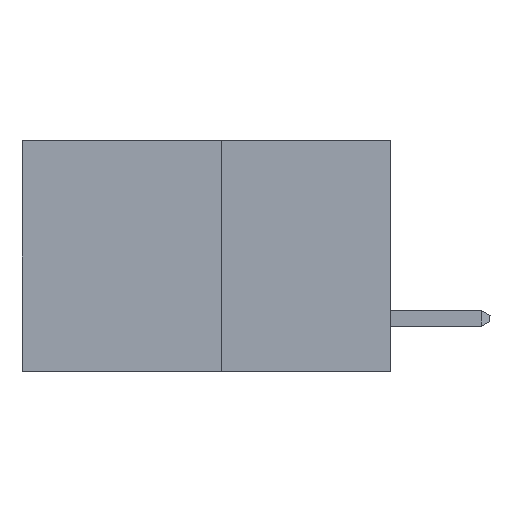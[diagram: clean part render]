
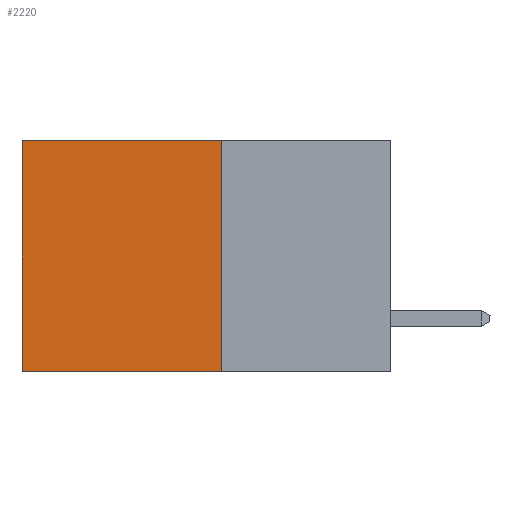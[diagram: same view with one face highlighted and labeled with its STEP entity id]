
A CAD part, left-side view. The second image highlights one B-rep face of the part: STEP entity #2220.
In plain terms, the highlighted planar face has unit normal (-1, 0, 0).
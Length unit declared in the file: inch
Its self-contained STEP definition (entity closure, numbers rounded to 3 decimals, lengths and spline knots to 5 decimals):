
#460 = DIRECTION ( 'NONE',  ( 1., 0., 0. ) ) ;
#852 = FACE_OUTER_BOUND ( 'NONE', #5256, .T. ) ;
#894 = EDGE_CURVE ( 'NONE', #5952, #5302, #2677, .T. ) ;
#1231 = CARTESIAN_POINT ( 'NONE',  ( 0.277, 0.59, -0.37 ) ) ;
#1289 = CARTESIAN_POINT ( 'NONE',  ( 0.277, 0.27, -0.37 ) ) ;
#1688 = EDGE_CURVE ( 'NONE', #5302, #4373, #8798, .T. ) ;
#1799 = ORIENTED_EDGE ( 'NONE', *, *, #894, .F. ) ;
#1964 = DIRECTION ( 'NONE',  ( 0., 1., 0. ) ) ;
#2111 = VECTOR ( 'NONE', #2915, 39.37008 ) ;
#2211 = CARTESIAN_POINT ( 'NONE',  ( 0.277, 0.27, 0. ) ) ;
#2220 = ADVANCED_FACE ( 'NONE', ( #852 ), #3283, .F. ) ;
#2549 = CARTESIAN_POINT ( 'NONE',  ( 0.277, 0.59, -0.37 ) ) ;
#2677 = LINE ( 'NONE', #3912, #8104 ) ;
#2915 = DIRECTION ( 'NONE',  ( 0., 1., 0. ) ) ;
#3283 = PLANE ( 'NONE',  #5911 ) ;
#3548 = VERTEX_POINT ( 'NONE', #8584 ) ;
#3601 = VECTOR ( 'NONE', #1964, 39.37008 ) ;
#3861 = CARTESIAN_POINT ( 'NONE',  ( 0.277, 0.27, -0.37 ) ) ;
#3912 = CARTESIAN_POINT ( 'NONE',  ( 0.277, 0.27, -0.37 ) ) ;
#4373 = VERTEX_POINT ( 'NONE', #1231 ) ;
#4508 = VECTOR ( 'NONE', #7494, 39.37008 ) ;
#5256 = EDGE_LOOP ( 'NONE', ( #8583, #7607, #1799, #7105 ) ) ;
#5302 = VERTEX_POINT ( 'NONE', #9095 ) ;
#5830 = LINE ( 'NONE', #2211, #2111 ) ;
#5911 = AXIS2_PLACEMENT_3D ( 'NONE', #1289, #460, #6773 ) ;
#5952 = VERTEX_POINT ( 'NONE', #8546 ) ;
#6773 = DIRECTION ( 'NONE',  ( 0., 0., -1. ) ) ;
#6848 = LINE ( 'NONE', #2549, #4508 ) ;
#7105 = ORIENTED_EDGE ( 'NONE', *, *, #8149, .T. ) ;
#7494 = DIRECTION ( 'NONE',  ( 0., 0., -1. ) ) ;
#7607 = ORIENTED_EDGE ( 'NONE', *, *, #1688, .F. ) ;
#7846 = EDGE_CURVE ( 'NONE', #3548, #4373, #6848, .T. ) ;
#8104 = VECTOR ( 'NONE', #8579, 39.37008 ) ;
#8149 = EDGE_CURVE ( 'NONE', #5952, #3548, #5830, .T. ) ;
#8546 = CARTESIAN_POINT ( 'NONE',  ( 0.277, 0.27, 0. ) ) ;
#8579 = DIRECTION ( 'NONE',  ( 0., 0., -1. ) ) ;
#8583 = ORIENTED_EDGE ( 'NONE', *, *, #7846, .T. ) ;
#8584 = CARTESIAN_POINT ( 'NONE',  ( 0.277, 0.59, 0. ) ) ;
#8798 = LINE ( 'NONE', #3861, #3601 ) ;
#9095 = CARTESIAN_POINT ( 'NONE',  ( 0.277, 0.27, -0.37 ) ) ;
